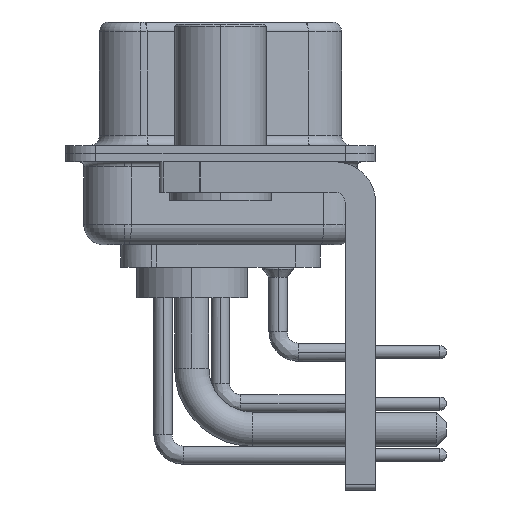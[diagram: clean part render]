
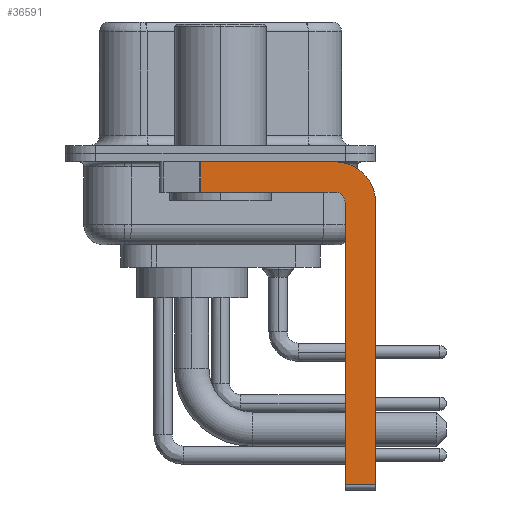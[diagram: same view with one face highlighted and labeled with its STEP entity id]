
A CAD part, left-side view. The second image highlights one B-rep face of the part: STEP entity #36591.
In plain terms, the highlighted planar face has unit normal (-1, 0, 0).
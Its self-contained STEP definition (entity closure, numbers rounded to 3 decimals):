
#156 = LINE ( 'NONE', #8675, #13973 ) ;
#449 = CARTESIAN_POINT ( 'NONE',  ( -2.9, -7.65, -2.4 ) ) ;
#697 = DIRECTION ( 'NONE',  ( 1., 0., 0. ) ) ;
#844 = CARTESIAN_POINT ( 'NONE',  ( -2.9, -7.65, -16.35 ) ) ;
#997 = EDGE_CURVE ( 'NONE', #16772, #24412, #7073, .T. ) ;
#1028 = CARTESIAN_POINT ( 'NONE',  ( -2.9, -5.65, -16.35 ) ) ;
#1430 = EDGE_CURVE ( 'NONE', #33099, #24412, #32502, .T. ) ;
#1739 = AXIS2_PLACEMENT_3D ( 'NONE', #17600, #697, #28551 ) ;
#2366 = DIRECTION ( 'NONE',  ( 0., 0., -1. ) ) ;
#2479 = CIRCLE ( 'NONE', #20325, 2. ) ;
#2793 = ORIENTED_EDGE ( 'NONE', *, *, #16784, .F. ) ;
#3526 = DIRECTION ( 'NONE',  ( 0., -1., 0. ) ) ;
#3572 = CARTESIAN_POINT ( 'NONE',  ( -2.9, 0.978, -0.4 ) ) ;
#4468 = DIRECTION ( 'NONE',  ( -1., 0., 0. ) ) ;
#5730 = ORIENTED_EDGE ( 'NONE', *, *, #26646, .F. ) ;
#6768 = LINE ( 'NONE', #1028, #6798 ) ;
#6798 = VECTOR ( 'NONE', #32059, 1000. ) ;
#7073 = LINE ( 'NONE', #24182, #18557 ) ;
#8358 = VERTEX_POINT ( 'NONE', #844 ) ;
#8675 = CARTESIAN_POINT ( 'NONE',  ( -2.9, -6.15, -16.6 ) ) ;
#10118 = ORIENTED_EDGE ( 'NONE', *, *, #18567, .F. ) ;
#11156 = ORIENTED_EDGE ( 'NONE', *, *, #23631, .F. ) ;
#11257 = PLANE ( 'NONE',  #1739 ) ;
#11278 = CARTESIAN_POINT ( 'NONE',  ( -2.9, -5.65, -2.4 ) ) ;
#11870 = LINE ( 'NONE', #23222, #30488 ) ;
#12292 = CARTESIAN_POINT ( 'NONE',  ( -2.9, -5.65, -0.4 ) ) ;
#13973 = VECTOR ( 'NONE', #34716, 1000. ) ;
#14129 = DIRECTION ( 'NONE',  ( 0., 0., -1. ) ) ;
#14437 = VERTEX_POINT ( 'NONE', #12292 ) ;
#16772 = VERTEX_POINT ( 'NONE', #25628 ) ;
#16784 = EDGE_CURVE ( 'NONE', #33099, #14437, #11870, .T. ) ;
#16874 = VERTEX_POINT ( 'NONE', #32675 ) ;
#17600 = CARTESIAN_POINT ( 'NONE',  ( -2.9, -5.65, -2.4 ) ) ;
#17772 = EDGE_CURVE ( 'NONE', #16874, #8358, #6768, .T. ) ;
#17810 = VERTEX_POINT ( 'NONE', #21098 ) ;
#18209 = DIRECTION ( 'NONE',  ( 0., 0., -1. ) ) ;
#18557 = VECTOR ( 'NONE', #21401, 1000. ) ;
#18567 = EDGE_CURVE ( 'NONE', #16874, #17810, #156, .T. ) ;
#19447 = ORIENTED_EDGE ( 'NONE', *, *, #17772, .T. ) ;
#19673 = DIRECTION ( 'NONE',  ( 1., 0., 0. ) ) ;
#20325 = AXIS2_PLACEMENT_3D ( 'NONE', #11278, #19673, #2366 ) ;
#21098 = CARTESIAN_POINT ( 'NONE',  ( -2.9, -6.15, -2.4 ) ) ;
#21401 = DIRECTION ( 'NONE',  ( 0., 1., 0. ) ) ;
#22314 = LINE ( 'NONE', #36255, #27217 ) ;
#23222 = CARTESIAN_POINT ( 'NONE',  ( -2.9, 3., -0.4 ) ) ;
#23631 = EDGE_CURVE ( 'NONE', #24694, #8358, #22314, .T. ) ;
#23798 = DIRECTION ( 'NONE',  ( 0., 0., 1. ) ) ;
#24143 = CARTESIAN_POINT ( 'NONE',  ( -2.9, 0.978, -1.9 ) ) ;
#24182 = CARTESIAN_POINT ( 'NONE',  ( -2.9, -5.65, -1.9 ) ) ;
#24412 = VERTEX_POINT ( 'NONE', #24616 ) ;
#24616 = CARTESIAN_POINT ( 'NONE',  ( -2.9, 0.978, -1.9 ) ) ;
#24694 = VERTEX_POINT ( 'NONE', #449 ) ;
#25575 = FACE_OUTER_BOUND ( 'NONE', #26758, .T. ) ;
#25628 = CARTESIAN_POINT ( 'NONE',  ( -2.9, -5.65, -1.9 ) ) ;
#26646 = EDGE_CURVE ( 'NONE', #14437, #24694, #2479, .T. ) ;
#26758 = EDGE_LOOP ( 'NONE', ( #2793, #33027, #35414, #30212, #10118, #19447, #11156, #5730 ) ) ;
#27217 = VECTOR ( 'NONE', #14129, 1000. ) ;
#28551 = DIRECTION ( 'NONE',  ( 0., 0., -1. ) ) ;
#30212 = ORIENTED_EDGE ( 'NONE', *, *, #30646, .F. ) ;
#30488 = VECTOR ( 'NONE', #3526, 1000. ) ;
#30646 = EDGE_CURVE ( 'NONE', #17810, #16772, #31738, .T. ) ;
#31738 = CIRCLE ( 'NONE', #32912, 0.5 ) ;
#31991 = CARTESIAN_POINT ( 'NONE',  ( -2.9, -5.65, -2.4 ) ) ;
#32059 = DIRECTION ( 'NONE',  ( 0., -1., 0. ) ) ;
#32502 = LINE ( 'NONE', #24143, #35307 ) ;
#32675 = CARTESIAN_POINT ( 'NONE',  ( -2.9, -6.15, -16.35 ) ) ;
#32912 = AXIS2_PLACEMENT_3D ( 'NONE', #31991, #4468, #23798 ) ;
#33027 = ORIENTED_EDGE ( 'NONE', *, *, #1430, .T. ) ;
#33099 = VERTEX_POINT ( 'NONE', #3572 ) ;
#34716 = DIRECTION ( 'NONE',  ( 0., 0., 1. ) ) ;
#35307 = VECTOR ( 'NONE', #18209, 1000. ) ;
#35414 = ORIENTED_EDGE ( 'NONE', *, *, #997, .F. ) ;
#36255 = CARTESIAN_POINT ( 'NONE',  ( -2.9, -7.65, -2.4 ) ) ;
#36591 = ADVANCED_FACE ( 'NONE', ( #25575 ), #11257, .F. ) ;
